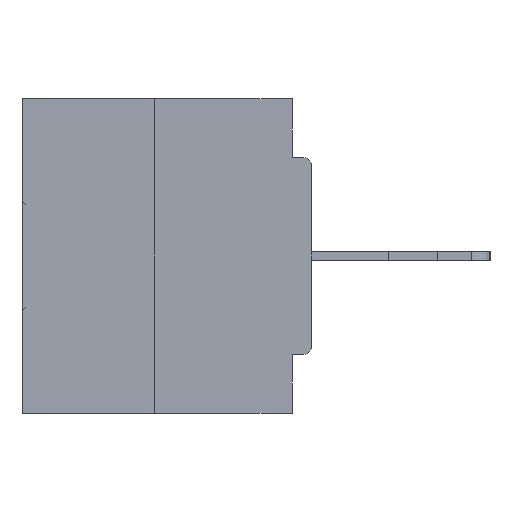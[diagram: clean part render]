
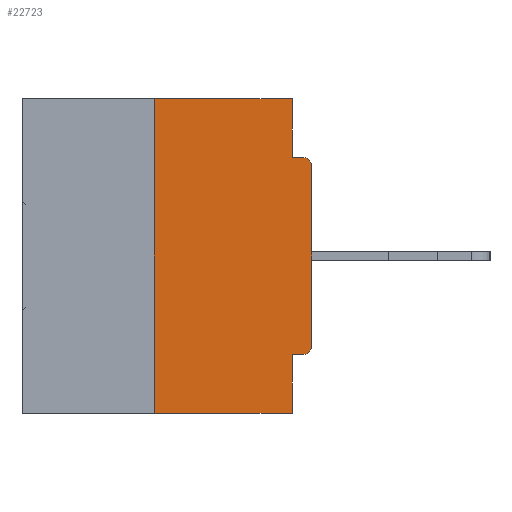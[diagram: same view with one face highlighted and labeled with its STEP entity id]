
A CAD part, left-side view. The second image highlights one B-rep face of the part: STEP entity #22723.
In plain terms, the highlighted planar face has unit normal (-1, 0, 0).
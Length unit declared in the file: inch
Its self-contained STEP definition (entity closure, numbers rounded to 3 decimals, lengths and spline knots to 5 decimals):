
#219 = CARTESIAN_POINT ( 'NONE',  ( 0., 0.031, -0.5 ) ) ;
#610 = CARTESIAN_POINT ( 'NONE',  ( 0., 0.031, -0.5 ) ) ;
#1395 = DIRECTION ( 'NONE',  ( 0., 0., -1. ) ) ;
#1544 = PLANE ( 'NONE',  #15827 ) ;
#2720 = EDGE_CURVE ( 'NONE', #24445, #35891, #9634, .T. ) ;
#3278 = DIRECTION ( 'NONE',  ( 0., 0., -1. ) ) ;
#3377 = DIRECTION ( 'NONE',  ( 0., 0., -1. ) ) ;
#3570 = CARTESIAN_POINT ( 'NONE',  ( 0., 0.25, -0.5 ) ) ;
#3642 = CARTESIAN_POINT ( 'NONE',  ( 0., 0.25, 0. ) ) ;
#3953 = VERTEX_POINT ( 'NONE', #24147 ) ;
#4801 = EDGE_CURVE ( 'NONE', #24086, #17315, #29027, .T. ) ;
#5156 = ORIENTED_EDGE ( 'NONE', *, *, #2720, .T. ) ;
#8309 = EDGE_CURVE ( 'NONE', #3953, #27712, #26171, .T. ) ;
#8358 = VECTOR ( 'NONE', #13594, 39.37008 ) ;
#8547 = LINE ( 'NONE', #31482, #19648 ) ;
#8574 = ORIENTED_EDGE ( 'NONE', *, *, #4801, .T. ) ;
#9407 = VECTOR ( 'NONE', #17740, 39.37008 ) ;
#9494 = EDGE_CURVE ( 'NONE', #25223, #21666, #19481, .T. ) ;
#9634 = CIRCLE ( 'NONE', #24663, 0.015 ) ;
#11408 = CARTESIAN_POINT ( 'NONE',  ( 0., 0., -0.3915 ) ) ;
#11844 = LINE ( 'NONE', #31190, #34977 ) ;
#12257 = LINE ( 'NONE', #25828, #36306 ) ;
#12359 = ORIENTED_EDGE ( 'NONE', *, *, #27647, .F. ) ;
#12471 = DIRECTION ( 'NONE',  ( -1., 0., 0. ) ) ;
#12845 = CARTESIAN_POINT ( 'NONE',  ( 0., 0.015, -0.1085 ) ) ;
#12877 = EDGE_CURVE ( 'NONE', #16886, #27712, #35034, .T. ) ;
#13594 = DIRECTION ( 'NONE',  ( 0., -1., 0. ) ) ;
#13611 = CARTESIAN_POINT ( 'NONE',  ( 0., 0.031, -0.0935 ) ) ;
#13837 = VECTOR ( 'NONE', #15286, 39.37008 ) ;
#13849 = EDGE_CURVE ( 'NONE', #24445, #3953, #11844, .T. ) ;
#14537 = FACE_OUTER_BOUND ( 'NONE', #24502, .T. ) ;
#14620 = CARTESIAN_POINT ( 'NONE',  ( 0., 0.46, 0. ) ) ;
#15286 = DIRECTION ( 'NONE',  ( 0., 0., 1. ) ) ;
#15297 = CARTESIAN_POINT ( 'NONE',  ( 0., 0.25, 0. ) ) ;
#15317 = CARTESIAN_POINT ( 'NONE',  ( 0., 0.015, -0.3915 ) ) ;
#15585 = CARTESIAN_POINT ( 'NONE',  ( 0., 0.46, 0. ) ) ;
#15827 = AXIS2_PLACEMENT_3D ( 'NONE', #15585, #35470, #18182 ) ;
#15992 = ORIENTED_EDGE ( 'NONE', *, *, #34440, .F. ) ;
#16441 = CARTESIAN_POINT ( 'NONE',  ( 0., 0.015, -0.4065 ) ) ;
#16886 = VERTEX_POINT ( 'NONE', #3570 ) ;
#16951 = LINE ( 'NONE', #29067, #9407 ) ;
#17272 = CARTESIAN_POINT ( 'NONE',  ( 0., 0.031, 0. ) ) ;
#17315 = VERTEX_POINT ( 'NONE', #29447 ) ;
#17699 = VECTOR ( 'NONE', #28266, 39.37008 ) ;
#17736 = ORIENTED_EDGE ( 'NONE', *, *, #13849, .F. ) ;
#17740 = DIRECTION ( 'NONE',  ( 0., 0., 1. ) ) ;
#18182 = DIRECTION ( 'NONE',  ( 0., 0., -1. ) ) ;
#19481 = LINE ( 'NONE', #14620, #17699 ) ;
#19648 = VECTOR ( 'NONE', #23391, 39.37008 ) ;
#20401 = EDGE_CURVE ( 'NONE', #35891, #24086, #16951, .T. ) ;
#21284 = DIRECTION ( 'NONE',  ( -1., 0., 0. ) ) ;
#21601 = AXIS2_PLACEMENT_3D ( 'NONE', #12845, #21284, #26862 ) ;
#21666 = VERTEX_POINT ( 'NONE', #17272 ) ;
#22002 = ORIENTED_EDGE ( 'NONE', *, *, #20401, .T. ) ;
#22037 = VERTEX_POINT ( 'NONE', #13611 ) ;
#22723 = ADVANCED_FACE ( 'NONE', ( #14537 ), #1544, .F. ) ;
#23123 = DIRECTION ( 'NONE',  ( 0., 1., 0. ) ) ;
#23391 = DIRECTION ( 'NONE',  ( 0., -1., 0. ) ) ;
#23791 = ORIENTED_EDGE ( 'NONE', *, *, #12877, .T. ) ;
#24086 = VERTEX_POINT ( 'NONE', #32766 ) ;
#24147 = CARTESIAN_POINT ( 'NONE',  ( 0., 0.031, -0.4065 ) ) ;
#24445 = VERTEX_POINT ( 'NONE', #16441 ) ;
#24502 = EDGE_LOOP ( 'NONE', ( #33242, #29032, #23791, #30471, #17736, #5156, #22002, #8574, #15992, #12359 ) ) ;
#24663 = AXIS2_PLACEMENT_3D ( 'NONE', #15317, #12471, #1395 ) ;
#25223 = VERTEX_POINT ( 'NONE', #15297 ) ;
#25828 = CARTESIAN_POINT ( 'NONE',  ( 0., 0.031, 0. ) ) ;
#26171 = LINE ( 'NONE', #610, #36892 ) ;
#26862 = DIRECTION ( 'NONE',  ( 0., 0., -1. ) ) ;
#27647 = EDGE_CURVE ( 'NONE', #21666, #22037, #12257, .T. ) ;
#27712 = VERTEX_POINT ( 'NONE', #219 ) ;
#28266 = DIRECTION ( 'NONE',  ( 0., -1., 0. ) ) ;
#29027 = CIRCLE ( 'NONE', #21601, 0.015 ) ;
#29032 = ORIENTED_EDGE ( 'NONE', *, *, #34840, .F. ) ;
#29067 = CARTESIAN_POINT ( 'NONE',  ( 0., 0., 0. ) ) ;
#29447 = CARTESIAN_POINT ( 'NONE',  ( 0., 0.015, -0.0935 ) ) ;
#30471 = ORIENTED_EDGE ( 'NONE', *, *, #8309, .F. ) ;
#30858 = CARTESIAN_POINT ( 'NONE',  ( 0., 0.46, -0.5 ) ) ;
#31190 = CARTESIAN_POINT ( 'NONE',  ( 0., 0., -0.4065 ) ) ;
#31482 = CARTESIAN_POINT ( 'NONE',  ( 0., 0., -0.0935 ) ) ;
#31655 = LINE ( 'NONE', #3642, #13837 ) ;
#32766 = CARTESIAN_POINT ( 'NONE',  ( 0., 0., -0.1085 ) ) ;
#33242 = ORIENTED_EDGE ( 'NONE', *, *, #9494, .F. ) ;
#34440 = EDGE_CURVE ( 'NONE', #22037, #17315, #8547, .T. ) ;
#34840 = EDGE_CURVE ( 'NONE', #16886, #25223, #31655, .T. ) ;
#34977 = VECTOR ( 'NONE', #23123, 39.37008 ) ;
#35034 = LINE ( 'NONE', #30858, #8358 ) ;
#35470 = DIRECTION ( 'NONE',  ( 1., 0., 0. ) ) ;
#35891 = VERTEX_POINT ( 'NONE', #11408 ) ;
#36306 = VECTOR ( 'NONE', #3377, 39.37008 ) ;
#36892 = VECTOR ( 'NONE', #3278, 39.37008 ) ;
